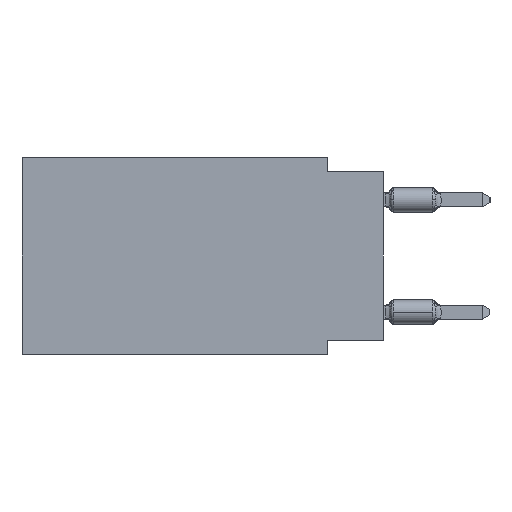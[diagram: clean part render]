
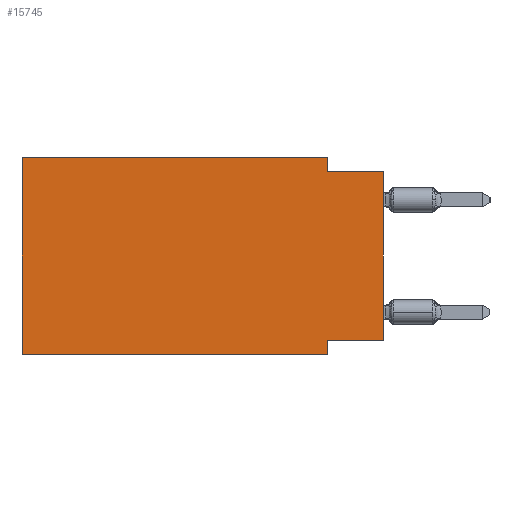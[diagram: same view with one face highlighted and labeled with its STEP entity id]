
A CAD part, left-side view. The second image highlights one B-rep face of the part: STEP entity #15745.
In plain terms, the highlighted planar face has unit normal (-1, 0, 0).
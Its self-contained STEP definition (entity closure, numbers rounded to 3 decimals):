
#174 = VERTEX_POINT ( 'NONE', #12568 ) ;
#572 = AXIS2_PLACEMENT_3D ( 'NONE', #41648, #2663, #19080 ) ;
#606 = LINE ( 'NONE', #4596, #36621 ) ;
#884 = DIRECTION ( 'NONE',  ( 0., -1., 0. ) ) ;
#1395 = VERTEX_POINT ( 'NONE', #12597 ) ;
#1435 = CARTESIAN_POINT ( 'NONE',  ( 0., 16.383, -8.89 ) ) ;
#1456 = ORIENTED_EDGE ( 'NONE', *, *, #22802, .F. ) ;
#1828 = CARTESIAN_POINT ( 'NONE',  ( 0., 2.54, 0. ) ) ;
#2663 = DIRECTION ( 'NONE',  ( 1., 0., 0. ) ) ;
#2696 = EDGE_CURVE ( 'NONE', #17060, #26740, #35414, .T. ) ;
#2872 = PLANE ( 'NONE',  #572 ) ;
#3234 = VECTOR ( 'NONE', #35281, 1000. ) ;
#3378 = CARTESIAN_POINT ( 'NONE',  ( 0., 2.54, -0.635 ) ) ;
#4143 = ORIENTED_EDGE ( 'NONE', *, *, #15871, .F. ) ;
#4223 = CARTESIAN_POINT ( 'NONE',  ( 0., 16.383, 0. ) ) ;
#4596 = CARTESIAN_POINT ( 'NONE',  ( 0., 2.54, -8.89 ) ) ;
#7392 = CARTESIAN_POINT ( 'NONE',  ( 0., 16.383, 0. ) ) ;
#7448 = CARTESIAN_POINT ( 'NONE',  ( 0., 16.383, 0. ) ) ;
#9543 = CARTESIAN_POINT ( 'NONE',  ( 0., 0., -8.255 ) ) ;
#10142 = ORIENTED_EDGE ( 'NONE', *, *, #32788, .F. ) ;
#11253 = CARTESIAN_POINT ( 'NONE',  ( 0., 0., 0. ) ) ;
#11951 = VERTEX_POINT ( 'NONE', #3378 ) ;
#12168 = ORIENTED_EDGE ( 'NONE', *, *, #37648, .F. ) ;
#12496 = EDGE_CURVE ( 'NONE', #23834, #29593, #17408, .T. ) ;
#12568 = CARTESIAN_POINT ( 'NONE',  ( 0., 2.54, -8.255 ) ) ;
#12597 = CARTESIAN_POINT ( 'NONE',  ( 0., 0., -0.635 ) ) ;
#13135 = ORIENTED_EDGE ( 'NONE', *, *, #36201, .T. ) ;
#13253 = CARTESIAN_POINT ( 'NONE',  ( 0., 16.383, -8.89 ) ) ;
#15745 = ADVANCED_FACE ( 'NONE', ( #41445 ), #2872, .F. ) ;
#15871 = EDGE_CURVE ( 'NONE', #11951, #1395, #26459, .T. ) ;
#16738 = CARTESIAN_POINT ( 'NONE',  ( 0., 0., -0.635 ) ) ;
#17041 = DIRECTION ( 'NONE',  ( 0., 0., 1. ) ) ;
#17060 = VERTEX_POINT ( 'NONE', #7448 ) ;
#17200 = DIRECTION ( 'NONE',  ( 0., 0., -1. ) ) ;
#17408 = LINE ( 'NONE', #1435, #18747 ) ;
#18695 = ORIENTED_EDGE ( 'NONE', *, *, #12496, .T. ) ;
#18747 = VECTOR ( 'NONE', #36587, 1000. ) ;
#19080 = DIRECTION ( 'NONE',  ( 0., 0., -1. ) ) ;
#19189 = CARTESIAN_POINT ( 'NONE',  ( 0., 2.54, 0. ) ) ;
#20842 = VERTEX_POINT ( 'NONE', #25189 ) ;
#22802 = EDGE_CURVE ( 'NONE', #26740, #11951, #39973, .T. ) ;
#22857 = DIRECTION ( 'NONE',  ( 0., 1., 0. ) ) ;
#22908 = EDGE_LOOP ( 'NONE', ( #13135, #4143, #1456, #29174, #10142, #18695, #32945, #12168 ) ) ;
#23834 = VERTEX_POINT ( 'NONE', #13253 ) ;
#24146 = DIRECTION ( 'NONE',  ( 0., 0., 1. ) ) ;
#24274 = VECTOR ( 'NONE', #27130, 1000. ) ;
#25189 = CARTESIAN_POINT ( 'NONE',  ( 0., 0., -8.255 ) ) ;
#26459 = LINE ( 'NONE', #16738, #3234 ) ;
#26555 = LINE ( 'NONE', #4223, #29140 ) ;
#26740 = VERTEX_POINT ( 'NONE', #19189 ) ;
#27130 = DIRECTION ( 'NONE',  ( 0., 0., -1. ) ) ;
#29140 = VECTOR ( 'NONE', #17041, 1000. ) ;
#29174 = ORIENTED_EDGE ( 'NONE', *, *, #2696, .F. ) ;
#29593 = VERTEX_POINT ( 'NONE', #32394 ) ;
#31485 = LINE ( 'NONE', #9543, #38154 ) ;
#32394 = CARTESIAN_POINT ( 'NONE',  ( 0., 2.54, -8.89 ) ) ;
#32788 = EDGE_CURVE ( 'NONE', #23834, #17060, #26555, .T. ) ;
#32945 = ORIENTED_EDGE ( 'NONE', *, *, #34338, .F. ) ;
#33221 = VECTOR ( 'NONE', #884, 1000. ) ;
#34338 = EDGE_CURVE ( 'NONE', #174, #29593, #606, .T. ) ;
#35281 = DIRECTION ( 'NONE',  ( 0., -1., 0. ) ) ;
#35414 = LINE ( 'NONE', #7392, #33221 ) ;
#36201 = EDGE_CURVE ( 'NONE', #20842, #1395, #40151, .T. ) ;
#36587 = DIRECTION ( 'NONE',  ( 0., -1., 0. ) ) ;
#36621 = VECTOR ( 'NONE', #17200, 1000. ) ;
#37648 = EDGE_CURVE ( 'NONE', #20842, #174, #31485, .T. ) ;
#38154 = VECTOR ( 'NONE', #22857, 1000. ) ;
#39439 = VECTOR ( 'NONE', #24146, 1000. ) ;
#39973 = LINE ( 'NONE', #1828, #24274 ) ;
#40151 = LINE ( 'NONE', #11253, #39439 ) ;
#41445 = FACE_OUTER_BOUND ( 'NONE', #22908, .T. ) ;
#41648 = CARTESIAN_POINT ( 'NONE',  ( 0., 16.383, 0. ) ) ;
